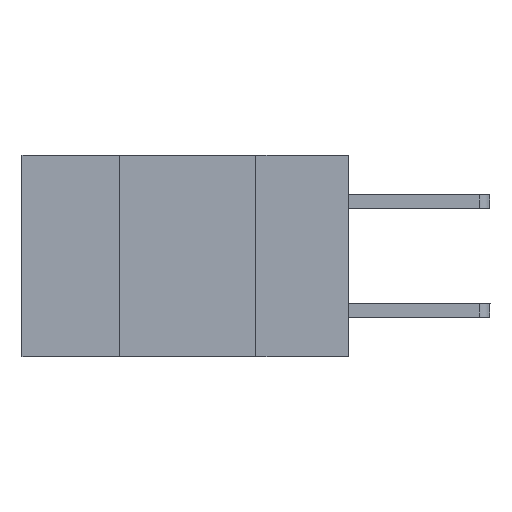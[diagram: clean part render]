
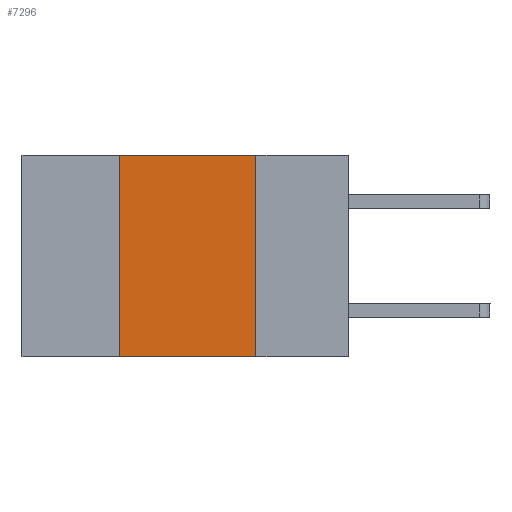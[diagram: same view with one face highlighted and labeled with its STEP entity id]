
A CAD part, left-side view. The second image highlights one B-rep face of the part: STEP entity #7296.
In plain terms, the highlighted planar face has unit normal (-1, 0, 0).
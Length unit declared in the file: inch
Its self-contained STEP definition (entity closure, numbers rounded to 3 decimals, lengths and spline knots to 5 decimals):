
#158 = DIRECTION ( 'NONE',  ( 0., 0., -1. ) ) ;
#667 = EDGE_CURVE ( 'NONE', #8220, #7670, #5934, .T. ) ;
#1953 = VECTOR ( 'NONE', #10761, 39.37008 ) ;
#2039 = ORIENTED_EDGE ( 'NONE', *, *, #6447, .T. ) ;
#2826 = VECTOR ( 'NONE', #9979, 39.37008 ) ;
#3100 = ORIENTED_EDGE ( 'NONE', *, *, #667, .F. ) ;
#3390 = EDGE_CURVE ( 'NONE', #7670, #8295, #7900, .T. ) ;
#3995 = VERTEX_POINT ( 'NONE', #4020 ) ;
#4020 = CARTESIAN_POINT ( 'NONE',  ( 0., 0.42, -0.37 ) ) ;
#4106 = CARTESIAN_POINT ( 'NONE',  ( 0., 0.17, -0.37 ) ) ;
#4378 = CARTESIAN_POINT ( 'NONE',  ( 0., 0.6, 0. ) ) ;
#4954 = FACE_OUTER_BOUND ( 'NONE', #10295, .T. ) ;
#5218 = DIRECTION ( 'NONE',  ( 1., 0., 0. ) ) ;
#5323 = LINE ( 'NONE', #8320, #2826 ) ;
#5546 = DIRECTION ( 'NONE',  ( 0., -1., 0. ) ) ;
#5934 = LINE ( 'NONE', #8836, #7622 ) ;
#6447 = EDGE_CURVE ( 'NONE', #3995, #8295, #8608, .T. ) ;
#6456 = ORIENTED_EDGE ( 'NONE', *, *, #9919, .F. ) ;
#6804 = ORIENTED_EDGE ( 'NONE', *, *, #3390, .F. ) ;
#7296 = ADVANCED_FACE ( 'NONE', ( #4954 ), #9361, .F. ) ;
#7453 = DIRECTION ( 'NONE',  ( 0., 0., -1. ) ) ;
#7622 = VECTOR ( 'NONE', #5546, 39.37008 ) ;
#7670 = VERTEX_POINT ( 'NONE', #9820 ) ;
#7900 = LINE ( 'NONE', #4106, #8160 ) ;
#8160 = VECTOR ( 'NONE', #7453, 39.37008 ) ;
#8220 = VERTEX_POINT ( 'NONE', #10470 ) ;
#8295 = VERTEX_POINT ( 'NONE', #8961 ) ;
#8320 = CARTESIAN_POINT ( 'NONE',  ( 0., 0.42, -0.37 ) ) ;
#8608 = LINE ( 'NONE', #9938, #1953 ) ;
#8836 = CARTESIAN_POINT ( 'NONE',  ( 0., 0.6, 0. ) ) ;
#8961 = CARTESIAN_POINT ( 'NONE',  ( 0., 0.17, -0.37 ) ) ;
#9361 = PLANE ( 'NONE',  #10628 ) ;
#9820 = CARTESIAN_POINT ( 'NONE',  ( 0., 0.17, 0. ) ) ;
#9919 = EDGE_CURVE ( 'NONE', #3995, #8220, #5323, .T. ) ;
#9938 = CARTESIAN_POINT ( 'NONE',  ( 0., 0.6, -0.37 ) ) ;
#9979 = DIRECTION ( 'NONE',  ( 0., 0., 1. ) ) ;
#10295 = EDGE_LOOP ( 'NONE', ( #6804, #3100, #6456, #2039 ) ) ;
#10470 = CARTESIAN_POINT ( 'NONE',  ( 0., 0.42, 0. ) ) ;
#10628 = AXIS2_PLACEMENT_3D ( 'NONE', #4378, #5218, #158 ) ;
#10761 = DIRECTION ( 'NONE',  ( 0., -1., 0. ) ) ;
